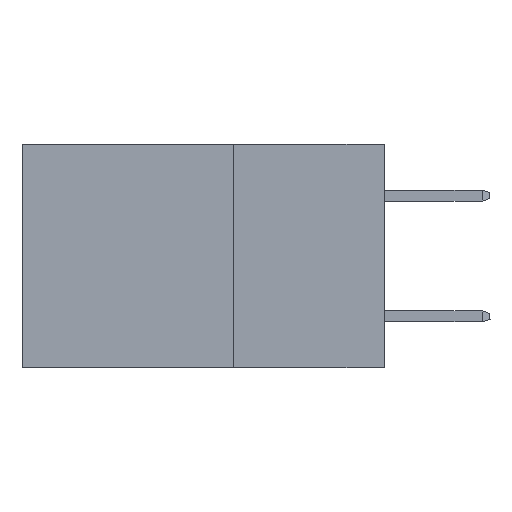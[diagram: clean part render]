
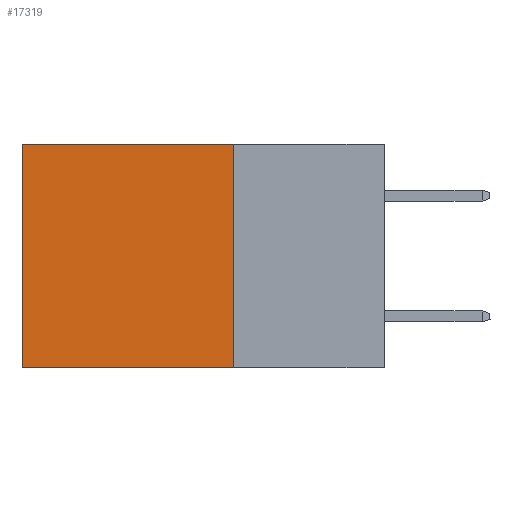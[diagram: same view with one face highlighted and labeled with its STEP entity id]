
A CAD part, left-side view. The second image highlights one B-rep face of the part: STEP entity #17319.
In plain terms, the highlighted planar face has unit normal (-1, 0, 0).
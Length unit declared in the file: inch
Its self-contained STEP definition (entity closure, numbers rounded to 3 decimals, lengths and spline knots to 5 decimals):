
#918 = FACE_OUTER_BOUND ( 'NONE', #6776, .T. ) ;
#1147 = CARTESIAN_POINT ( 'NONE',  ( 0.2615, 0.25, -0.37 ) ) ;
#2094 = CARTESIAN_POINT ( 'NONE',  ( 0.2615, 0.6, 0. ) ) ;
#2193 = EDGE_CURVE ( 'NONE', #13341, #16698, #14930, .T. ) ;
#3594 = DIRECTION ( 'NONE',  ( 0., 0., -1. ) ) ;
#5004 = CARTESIAN_POINT ( 'NONE',  ( 0.2615, 0.25, 0. ) ) ;
#5327 = VERTEX_POINT ( 'NONE', #2094 ) ;
#6776 = EDGE_LOOP ( 'NONE', ( #13063, #15654, #15520, #19533 ) ) ;
#7214 = VECTOR ( 'NONE', #17849, 39.37008 ) ;
#7451 = VECTOR ( 'NONE', #14939, 39.37008 ) ;
#7712 = CARTESIAN_POINT ( 'NONE',  ( 0.2615, 0.25, -0.37 ) ) ;
#8695 = CARTESIAN_POINT ( 'NONE',  ( 0.2615, 0.6, -0.37 ) ) ;
#8841 = LINE ( 'NONE', #8695, #16512 ) ;
#9282 = DIRECTION ( 'NONE',  ( 0., 0., -1. ) ) ;
#10251 = DIRECTION ( 'NONE',  ( 0., 0., -1. ) ) ;
#11954 = EDGE_CURVE ( 'NONE', #5327, #16698, #8841, .T. ) ;
#12444 = LINE ( 'NONE', #17444, #12952 ) ;
#12952 = VECTOR ( 'NONE', #3594, 39.37008 ) ;
#13063 = ORIENTED_EDGE ( 'NONE', *, *, #11954, .T. ) ;
#13341 = VERTEX_POINT ( 'NONE', #1147 ) ;
#13433 = CARTESIAN_POINT ( 'NONE',  ( 0.2615, 0.25, 0. ) ) ;
#14016 = CARTESIAN_POINT ( 'NONE',  ( 0.2615, 0.6, -0.37 ) ) ;
#14930 = LINE ( 'NONE', #19373, #7214 ) ;
#14939 = DIRECTION ( 'NONE',  ( 0., 1., 0. ) ) ;
#15371 = PLANE ( 'NONE',  #17553 ) ;
#15520 = ORIENTED_EDGE ( 'NONE', *, *, #19584, .F. ) ;
#15654 = ORIENTED_EDGE ( 'NONE', *, *, #2193, .F. ) ;
#16107 = VERTEX_POINT ( 'NONE', #5004 ) ;
#16512 = VECTOR ( 'NONE', #10251, 39.37008 ) ;
#16698 = VERTEX_POINT ( 'NONE', #14016 ) ;
#17319 = ADVANCED_FACE ( 'NONE', ( #918 ), #15371, .F. ) ;
#17444 = CARTESIAN_POINT ( 'NONE',  ( 0.2615, 0.25, -0.37 ) ) ;
#17553 = AXIS2_PLACEMENT_3D ( 'NONE', #7712, #18447, #9282 ) ;
#17849 = DIRECTION ( 'NONE',  ( 0., 1., 0. ) ) ;
#17861 = EDGE_CURVE ( 'NONE', #16107, #5327, #19678, .T. ) ;
#18447 = DIRECTION ( 'NONE',  ( 1., 0., 0. ) ) ;
#19373 = CARTESIAN_POINT ( 'NONE',  ( 0.2615, 0.25, -0.37 ) ) ;
#19533 = ORIENTED_EDGE ( 'NONE', *, *, #17861, .T. ) ;
#19584 = EDGE_CURVE ( 'NONE', #16107, #13341, #12444, .T. ) ;
#19678 = LINE ( 'NONE', #13433, #7451 ) ;
